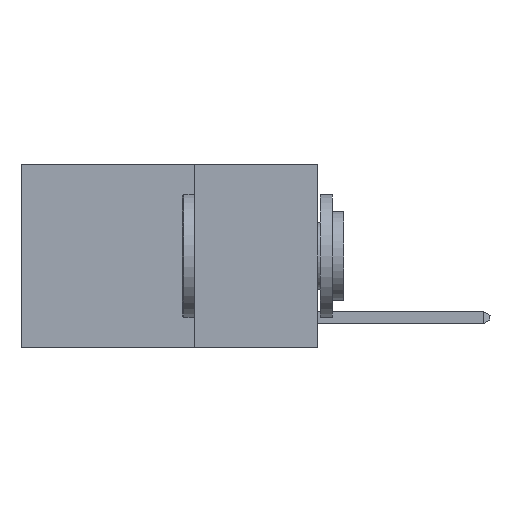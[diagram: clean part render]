
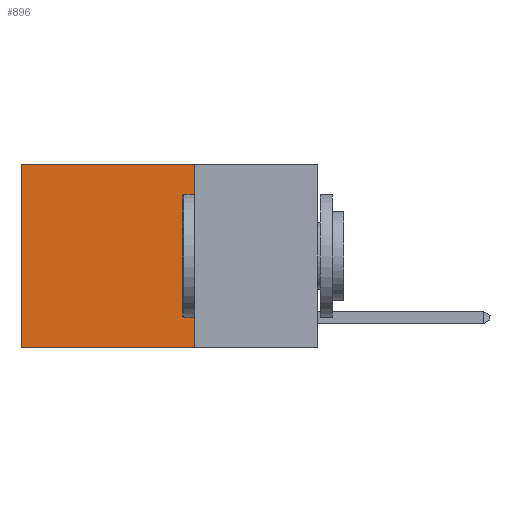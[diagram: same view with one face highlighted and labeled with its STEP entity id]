
A CAD part, left-side view. The second image highlights one B-rep face of the part: STEP entity #896.
In plain terms, the highlighted planar face has unit normal (-1, 0, 0).
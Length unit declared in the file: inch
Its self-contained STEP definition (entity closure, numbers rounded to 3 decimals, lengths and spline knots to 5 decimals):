
#896 = ADVANCED_FACE ( 'NONE', ( #12364 ), #5764, .F. ) ;
#1505 = CARTESIAN_POINT ( 'NONE',  ( 0.2625, 0.6, 0. ) ) ;
#2049 = CARTESIAN_POINT ( 'NONE',  ( 0.2625, 0.25, -0.37 ) ) ;
#3063 = LINE ( 'NONE', #12820, #13573 ) ;
#3144 = DIRECTION ( 'NONE',  ( 0., 1., 0. ) ) ;
#3202 = ORIENTED_EDGE ( 'NONE', *, *, #6242, .T. ) ;
#3308 = EDGE_CURVE ( 'NONE', #6052, #3792, #12700, .T. ) ;
#3514 = LINE ( 'NONE', #8648, #8755 ) ;
#3698 = EDGE_CURVE ( 'NONE', #5138, #6052, #3063, .T. ) ;
#3785 = DIRECTION ( 'NONE',  ( 0., 0., -1. ) ) ;
#3792 = VERTEX_POINT ( 'NONE', #9009 ) ;
#3948 = CARTESIAN_POINT ( 'NONE',  ( 0.2625, 0.6, 0. ) ) ;
#4097 = CARTESIAN_POINT ( 'NONE',  ( 0.2625, 0.25, 0. ) ) ;
#4573 = VECTOR ( 'NONE', #3144, 39.37008 ) ;
#4803 = VECTOR ( 'NONE', #7978, 39.37008 ) ;
#4810 = DIRECTION ( 'NONE',  ( 1., 0., 0. ) ) ;
#5138 = VERTEX_POINT ( 'NONE', #4097 ) ;
#5597 = CARTESIAN_POINT ( 'NONE',  ( 0.2625, 0.25, 0. ) ) ;
#5696 = ORIENTED_EDGE ( 'NONE', *, *, #13365, .T. ) ;
#5764 = PLANE ( 'NONE',  #8527 ) ;
#6052 = VERTEX_POINT ( 'NONE', #10406 ) ;
#6242 = EDGE_CURVE ( 'NONE', #5138, #8557, #3514, .T. ) ;
#6709 = EDGE_LOOP ( 'NONE', ( #5696, #8460, #11177, #3202 ) ) ;
#7574 = LINE ( 'NONE', #1505, #4803 ) ;
#7978 = DIRECTION ( 'NONE',  ( 0., 0., -1. ) ) ;
#8460 = ORIENTED_EDGE ( 'NONE', *, *, #3308, .F. ) ;
#8527 = AXIS2_PLACEMENT_3D ( 'NONE', #5597, #4810, #3785 ) ;
#8557 = VERTEX_POINT ( 'NONE', #3948 ) ;
#8648 = CARTESIAN_POINT ( 'NONE',  ( 0.2625, 0.25, 0. ) ) ;
#8755 = VECTOR ( 'NONE', #9686, 39.37008 ) ;
#9009 = CARTESIAN_POINT ( 'NONE',  ( 0.2625, 0.6, -0.37 ) ) ;
#9686 = DIRECTION ( 'NONE',  ( 0., 1., 0. ) ) ;
#9905 = DIRECTION ( 'NONE',  ( 0., 0., -1. ) ) ;
#10406 = CARTESIAN_POINT ( 'NONE',  ( 0.2625, 0.25, -0.37 ) ) ;
#11177 = ORIENTED_EDGE ( 'NONE', *, *, #3698, .F. ) ;
#12364 = FACE_OUTER_BOUND ( 'NONE', #6709, .T. ) ;
#12700 = LINE ( 'NONE', #2049, #4573 ) ;
#12820 = CARTESIAN_POINT ( 'NONE',  ( 0.2625, 0.25, 0. ) ) ;
#13365 = EDGE_CURVE ( 'NONE', #8557, #3792, #7574, .T. ) ;
#13573 = VECTOR ( 'NONE', #9905, 39.37008 ) ;
